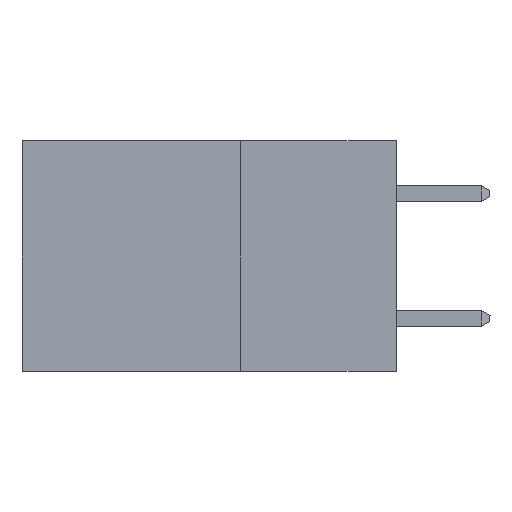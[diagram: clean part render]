
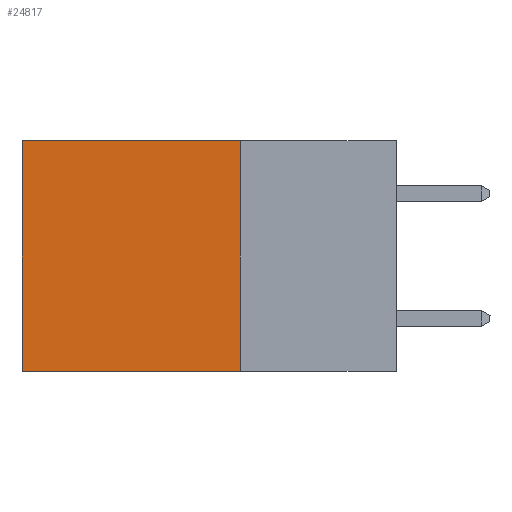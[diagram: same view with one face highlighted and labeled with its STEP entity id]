
A CAD part, left-side view. The second image highlights one B-rep face of the part: STEP entity #24817.
In plain terms, the highlighted planar face has unit normal (-1, 0, 0).
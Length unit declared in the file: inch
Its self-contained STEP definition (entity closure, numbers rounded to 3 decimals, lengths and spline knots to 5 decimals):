
#100 = CARTESIAN_POINT ( 'NONE',  ( 0.2615, 0.25, 0. ) ) ;
#449 = VERTEX_POINT ( 'NONE', #10161 ) ;
#477 = EDGE_CURVE ( 'NONE', #16727, #6720, #13359, .T. ) ;
#984 = ORIENTED_EDGE ( 'NONE', *, *, #1044, .F. ) ;
#1044 = EDGE_CURVE ( 'NONE', #449, #6720, #8769, .T. ) ;
#2654 = DIRECTION ( 'NONE',  ( 0., 0., -1. ) ) ;
#3864 = PLANE ( 'NONE',  #10589 ) ;
#5431 = EDGE_LOOP ( 'NONE', ( #6188, #984, #19095, #22957 ) ) ;
#5900 = DIRECTION ( 'NONE',  ( 1., 0., 0. ) ) ;
#6188 = ORIENTED_EDGE ( 'NONE', *, *, #477, .T. ) ;
#6613 = DIRECTION ( 'NONE',  ( 0., 0., -1. ) ) ;
#6698 = VECTOR ( 'NONE', #23465, 39.37008 ) ;
#6720 = VERTEX_POINT ( 'NONE', #7078 ) ;
#7078 = CARTESIAN_POINT ( 'NONE',  ( 0.2615, 0.6, -0.37 ) ) ;
#7533 = VECTOR ( 'NONE', #24023, 39.37008 ) ;
#7849 = CARTESIAN_POINT ( 'NONE',  ( 0.2615, 0.25, -0.37 ) ) ;
#8467 = CARTESIAN_POINT ( 'NONE',  ( 0.2615, 0.6, 0. ) ) ;
#8769 = LINE ( 'NONE', #17968, #7533 ) ;
#10161 = CARTESIAN_POINT ( 'NONE',  ( 0.2615, 0.25, -0.37 ) ) ;
#10589 = AXIS2_PLACEMENT_3D ( 'NONE', #7849, #5900, #19920 ) ;
#11095 = EDGE_CURVE ( 'NONE', #24922, #16727, #12020, .T. ) ;
#11584 = VECTOR ( 'NONE', #6613, 39.37008 ) ;
#12020 = LINE ( 'NONE', #21470, #6698 ) ;
#13359 = LINE ( 'NONE', #19780, #23375 ) ;
#16727 = VERTEX_POINT ( 'NONE', #8467 ) ;
#17968 = CARTESIAN_POINT ( 'NONE',  ( 0.2615, 0.25, -0.37 ) ) ;
#18596 = CARTESIAN_POINT ( 'NONE',  ( 0.2615, 0.25, -0.37 ) ) ;
#19095 = ORIENTED_EDGE ( 'NONE', *, *, #25043, .F. ) ;
#19780 = CARTESIAN_POINT ( 'NONE',  ( 0.2615, 0.6, -0.37 ) ) ;
#19920 = DIRECTION ( 'NONE',  ( 0., 0., -1. ) ) ;
#21470 = CARTESIAN_POINT ( 'NONE',  ( 0.2615, 0.25, 0. ) ) ;
#22229 = LINE ( 'NONE', #18596, #11584 ) ;
#22556 = FACE_OUTER_BOUND ( 'NONE', #5431, .T. ) ;
#22957 = ORIENTED_EDGE ( 'NONE', *, *, #11095, .T. ) ;
#23375 = VECTOR ( 'NONE', #2654, 39.37008 ) ;
#23465 = DIRECTION ( 'NONE',  ( 0., 1., 0. ) ) ;
#24023 = DIRECTION ( 'NONE',  ( 0., 1., 0. ) ) ;
#24817 = ADVANCED_FACE ( 'NONE', ( #22556 ), #3864, .F. ) ;
#24922 = VERTEX_POINT ( 'NONE', #100 ) ;
#25043 = EDGE_CURVE ( 'NONE', #24922, #449, #22229, .T. ) ;
